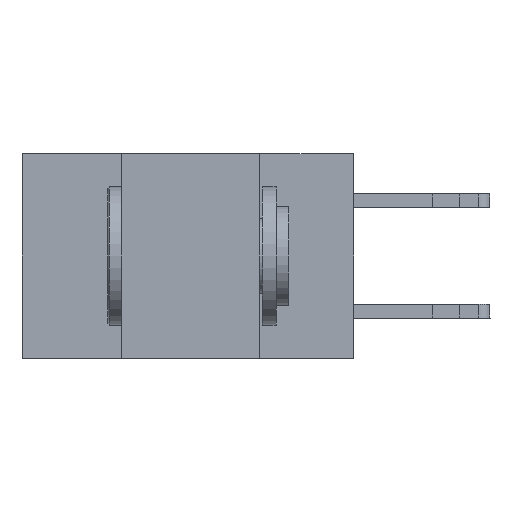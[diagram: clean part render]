
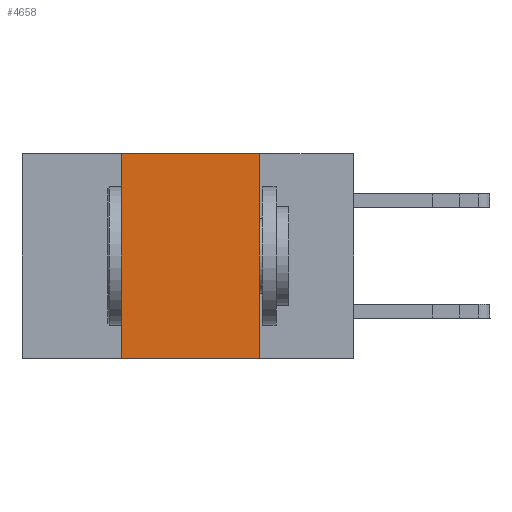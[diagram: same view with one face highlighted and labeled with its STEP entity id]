
A CAD part, left-side view. The second image highlights one B-rep face of the part: STEP entity #4658.
In plain terms, the highlighted planar face has unit normal (-1, 0, 0).
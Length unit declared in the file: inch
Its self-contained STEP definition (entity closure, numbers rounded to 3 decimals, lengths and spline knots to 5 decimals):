
#20 = DIRECTION ( 'NONE',  ( 1., 0., 0. ) ) ;
#893 = DIRECTION ( 'NONE',  ( 0., 0., 1. ) ) ;
#1779 = LINE ( 'NONE', #20072, #10094 ) ;
#2143 = CARTESIAN_POINT ( 'NONE',  ( 0., 0.17, 0. ) ) ;
#2405 = EDGE_CURVE ( 'NONE', #15517, #17441, #26331, .T. ) ;
#2539 = CARTESIAN_POINT ( 'NONE',  ( 0., 0.42, 0. ) ) ;
#2713 = VECTOR ( 'NONE', #8801, 39.37008 ) ;
#4658 = ADVANCED_FACE ( 'NONE', ( #9879 ), #26365, .F. ) ;
#6129 = CARTESIAN_POINT ( 'NONE',  ( 0., 0.6, 0. ) ) ;
#7209 = VERTEX_POINT ( 'NONE', #14984 ) ;
#7879 = ORIENTED_EDGE ( 'NONE', *, *, #22950, .F. ) ;
#8176 = DIRECTION ( 'NONE',  ( 0., 0., -1. ) ) ;
#8801 = DIRECTION ( 'NONE',  ( 0., -1., 0. ) ) ;
#9879 = FACE_OUTER_BOUND ( 'NONE', #23235, .T. ) ;
#10094 = VECTOR ( 'NONE', #16017, 39.37008 ) ;
#12762 = DIRECTION ( 'NONE',  ( 0., -1., 0. ) ) ;
#13507 = VECTOR ( 'NONE', #893, 39.37008 ) ;
#13626 = LINE ( 'NONE', #17123, #2713 ) ;
#14584 = LINE ( 'NONE', #22952, #20393 ) ;
#14984 = CARTESIAN_POINT ( 'NONE',  ( 0., 0.17, -0.37 ) ) ;
#15469 = VERTEX_POINT ( 'NONE', #2143 ) ;
#15517 = VERTEX_POINT ( 'NONE', #21737 ) ;
#16017 = DIRECTION ( 'NONE',  ( 0., 0., -1. ) ) ;
#17123 = CARTESIAN_POINT ( 'NONE',  ( 0., 0.6, -0.37 ) ) ;
#17398 = ORIENTED_EDGE ( 'NONE', *, *, #25394, .T. ) ;
#17441 = VERTEX_POINT ( 'NONE', #2539 ) ;
#20072 = CARTESIAN_POINT ( 'NONE',  ( 0., 0.17, 0. ) ) ;
#20241 = ORIENTED_EDGE ( 'NONE', *, *, #22738, .F. ) ;
#20393 = VECTOR ( 'NONE', #12762, 39.37008 ) ;
#21737 = CARTESIAN_POINT ( 'NONE',  ( 0., 0.42, -0.37 ) ) ;
#22738 = EDGE_CURVE ( 'NONE', #15469, #7209, #1779, .T. ) ;
#22950 = EDGE_CURVE ( 'NONE', #17441, #15469, #14584, .T. ) ;
#22952 = CARTESIAN_POINT ( 'NONE',  ( 0., 0.6, 0. ) ) ;
#23235 = EDGE_LOOP ( 'NONE', ( #20241, #7879, #24227, #17398 ) ) ;
#23418 = CARTESIAN_POINT ( 'NONE',  ( 0., 0.42, 0. ) ) ;
#24227 = ORIENTED_EDGE ( 'NONE', *, *, #2405, .F. ) ;
#24926 = AXIS2_PLACEMENT_3D ( 'NONE', #6129, #20, #8176 ) ;
#25394 = EDGE_CURVE ( 'NONE', #15517, #7209, #13626, .T. ) ;
#26331 = LINE ( 'NONE', #23418, #13507 ) ;
#26365 = PLANE ( 'NONE',  #24926 ) ;
